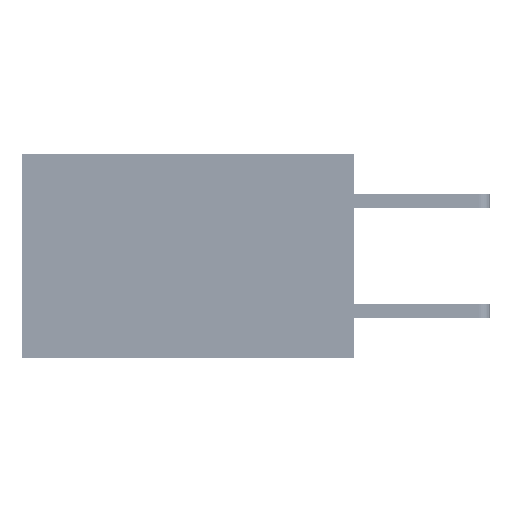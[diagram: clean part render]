
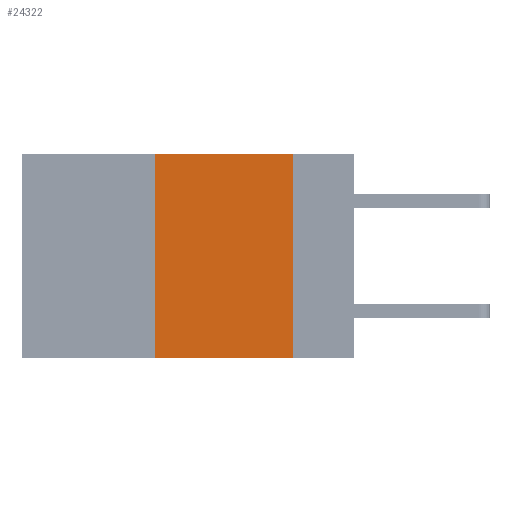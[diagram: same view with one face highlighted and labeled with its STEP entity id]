
A CAD part, left-side view. The second image highlights one B-rep face of the part: STEP entity #24322.
In plain terms, the highlighted planar face has unit normal (-1, 0, 0).
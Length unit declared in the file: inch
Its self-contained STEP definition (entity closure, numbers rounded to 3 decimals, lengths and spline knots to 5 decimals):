
#901 = EDGE_CURVE ( 'NONE', #27928, #6454, #31794, .T. ) ;
#6454 = VERTEX_POINT ( 'NONE', #16507 ) ;
#6941 = LINE ( 'NONE', #38697, #10823 ) ;
#7242 = CARTESIAN_POINT ( 'NONE',  ( 0., 0.6, -0.37 ) ) ;
#7725 = VERTEX_POINT ( 'NONE', #17800 ) ;
#7947 = DIRECTION ( 'NONE',  ( 0., -1., 0. ) ) ;
#8716 = CARTESIAN_POINT ( 'NONE',  ( 0., 0.11, 0. ) ) ;
#10124 = FACE_OUTER_BOUND ( 'NONE', #27569, .T. ) ;
#10417 = EDGE_CURVE ( 'NONE', #28614, #7725, #17131, .T. ) ;
#10823 = VECTOR ( 'NONE', #7947, 39.37008 ) ;
#16507 = CARTESIAN_POINT ( 'NONE',  ( 0., 0.11, -0.37 ) ) ;
#17131 = LINE ( 'NONE', #35771, #34117 ) ;
#17800 = CARTESIAN_POINT ( 'NONE',  ( 0., 0.36, 0. ) ) ;
#19198 = ORIENTED_EDGE ( 'NONE', *, *, #10417, .F. ) ;
#21447 = VECTOR ( 'NONE', #26650, 39.37008 ) ;
#23775 = CARTESIAN_POINT ( 'NONE',  ( 0., 0.11, 0. ) ) ;
#24322 = ADVANCED_FACE ( 'NONE', ( #10124 ), #45272, .F. ) ;
#24906 = DIRECTION ( 'NONE',  ( 0., 0., 1. ) ) ;
#25376 = DIRECTION ( 'NONE',  ( 1., 0., 0. ) ) ;
#26204 = ORIENTED_EDGE ( 'NONE', *, *, #901, .F. ) ;
#26650 = DIRECTION ( 'NONE',  ( 0., 0., -1. ) ) ;
#27569 = EDGE_LOOP ( 'NONE', ( #26204, #33824, #19198, #30229 ) ) ;
#27928 = VERTEX_POINT ( 'NONE', #8716 ) ;
#28614 = VERTEX_POINT ( 'NONE', #31600 ) ;
#30229 = ORIENTED_EDGE ( 'NONE', *, *, #41029, .T. ) ;
#31600 = CARTESIAN_POINT ( 'NONE',  ( 0., 0.36, -0.37 ) ) ;
#31794 = LINE ( 'NONE', #23775, #21447 ) ;
#32544 = VECTOR ( 'NONE', #34363, 39.37008 ) ;
#33824 = ORIENTED_EDGE ( 'NONE', *, *, #37081, .F. ) ;
#34117 = VECTOR ( 'NONE', #24906, 39.37008 ) ;
#34363 = DIRECTION ( 'NONE',  ( 0., -1., 0. ) ) ;
#35771 = CARTESIAN_POINT ( 'NONE',  ( 0., 0.36, 0. ) ) ;
#37081 = EDGE_CURVE ( 'NONE', #7725, #27928, #6941, .T. ) ;
#37757 = CARTESIAN_POINT ( 'NONE',  ( 0., 0.6, 0. ) ) ;
#38697 = CARTESIAN_POINT ( 'NONE',  ( 0., 0.6, 0. ) ) ;
#41029 = EDGE_CURVE ( 'NONE', #28614, #6454, #42112, .T. ) ;
#42112 = LINE ( 'NONE', #7242, #32544 ) ;
#45272 = PLANE ( 'NONE',  #50995 ) ;
#45521 = DIRECTION ( 'NONE',  ( 0., 0., -1. ) ) ;
#50995 = AXIS2_PLACEMENT_3D ( 'NONE', #37757, #25376, #45521 ) ;
